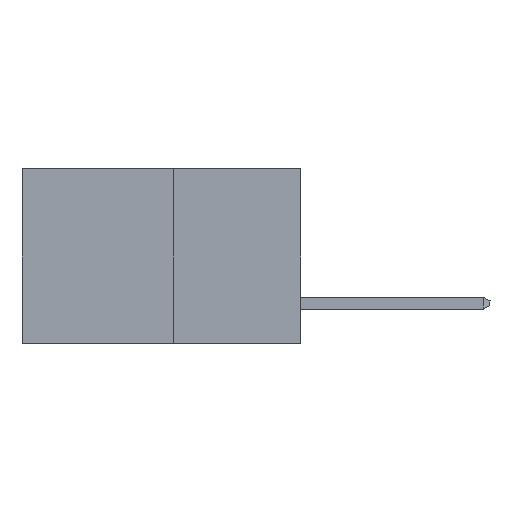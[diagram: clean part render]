
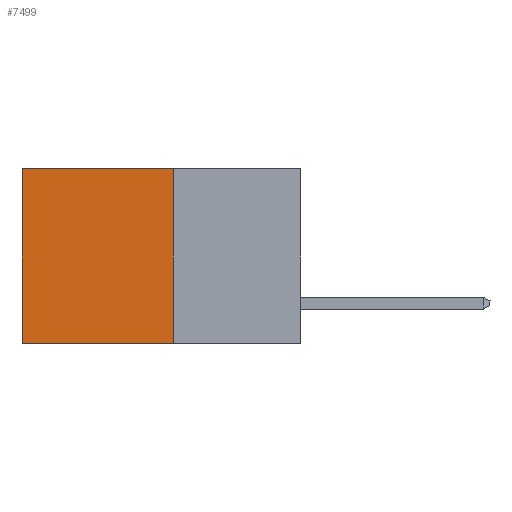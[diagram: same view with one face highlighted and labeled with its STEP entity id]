
A CAD part, left-side view. The second image highlights one B-rep face of the part: STEP entity #7499.
In plain terms, the highlighted planar face has unit normal (-1, 0, 0).
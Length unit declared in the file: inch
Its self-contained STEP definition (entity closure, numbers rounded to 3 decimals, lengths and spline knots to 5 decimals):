
#807 = PLANE ( 'NONE',  #13273 ) ;
#880 = EDGE_CURVE ( 'NONE', #15469, #11598, #9581, .T. ) ;
#2018 = CARTESIAN_POINT ( 'NONE',  ( 0.277, 0.27, -0.37 ) ) ;
#2328 = VERTEX_POINT ( 'NONE', #10864 ) ;
#2412 = FACE_OUTER_BOUND ( 'NONE', #15358, .T. ) ;
#2850 = CARTESIAN_POINT ( 'NONE',  ( 0.277, 0.59, -0.37 ) ) ;
#3269 = DIRECTION ( 'NONE',  ( 1., 0., 0. ) ) ;
#3621 = VECTOR ( 'NONE', #12631, 39.37008 ) ;
#4250 = VECTOR ( 'NONE', #7110, 39.37008 ) ;
#4430 = VECTOR ( 'NONE', #7455, 39.37008 ) ;
#4452 = ORIENTED_EDGE ( 'NONE', *, *, #880, .F. ) ;
#4778 = ORIENTED_EDGE ( 'NONE', *, *, #9023, .T. ) ;
#5201 = EDGE_CURVE ( 'NONE', #11598, #11370, #12855, .T. ) ;
#5622 = CARTESIAN_POINT ( 'NONE',  ( 0.277, 0.27, -0.37 ) ) ;
#7110 = DIRECTION ( 'NONE',  ( 0., 0., -1. ) ) ;
#7247 = CARTESIAN_POINT ( 'NONE',  ( 0.277, 0.27, -0.37 ) ) ;
#7388 = CARTESIAN_POINT ( 'NONE',  ( 0.277, 0.27, -0.37 ) ) ;
#7455 = DIRECTION ( 'NONE',  ( 0., 1., 0. ) ) ;
#7457 = LINE ( 'NONE', #15416, #4250 ) ;
#7499 = ADVANCED_FACE ( 'NONE', ( #2412 ), #807, .F. ) ;
#8589 = CARTESIAN_POINT ( 'NONE',  ( 0.277, 0.27, 0. ) ) ;
#8817 = EDGE_CURVE ( 'NONE', #2328, #11370, #7457, .T. ) ;
#9023 = EDGE_CURVE ( 'NONE', #15469, #2328, #14322, .T. ) ;
#9581 = LINE ( 'NONE', #7388, #3621 ) ;
#10028 = VECTOR ( 'NONE', #15326, 39.37008 ) ;
#10583 = CARTESIAN_POINT ( 'NONE',  ( 0.277, 0.27, 0. ) ) ;
#10864 = CARTESIAN_POINT ( 'NONE',  ( 0.277, 0.59, 0. ) ) ;
#11370 = VERTEX_POINT ( 'NONE', #2850 ) ;
#11598 = VERTEX_POINT ( 'NONE', #5622 ) ;
#11655 = DIRECTION ( 'NONE',  ( 0., 0., -1. ) ) ;
#12631 = DIRECTION ( 'NONE',  ( 0., 0., -1. ) ) ;
#12855 = LINE ( 'NONE', #7247, #10028 ) ;
#13273 = AXIS2_PLACEMENT_3D ( 'NONE', #2018, #3269, #11655 ) ;
#13899 = ORIENTED_EDGE ( 'NONE', *, *, #8817, .T. ) ;
#14322 = LINE ( 'NONE', #8589, #4430 ) ;
#15320 = ORIENTED_EDGE ( 'NONE', *, *, #5201, .F. ) ;
#15326 = DIRECTION ( 'NONE',  ( 0., 1., 0. ) ) ;
#15358 = EDGE_LOOP ( 'NONE', ( #13899, #15320, #4452, #4778 ) ) ;
#15416 = CARTESIAN_POINT ( 'NONE',  ( 0.277, 0.59, -0.37 ) ) ;
#15469 = VERTEX_POINT ( 'NONE', #10583 ) ;
